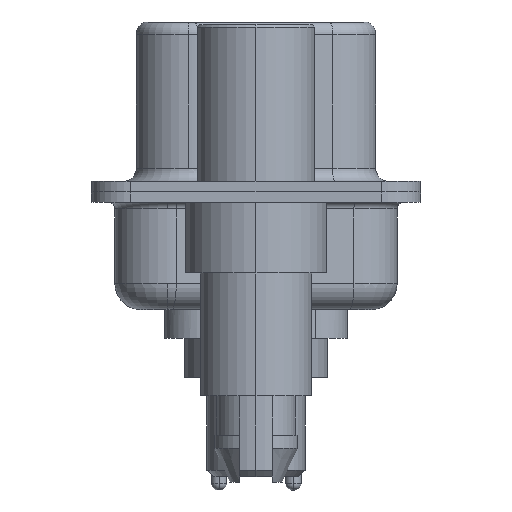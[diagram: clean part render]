
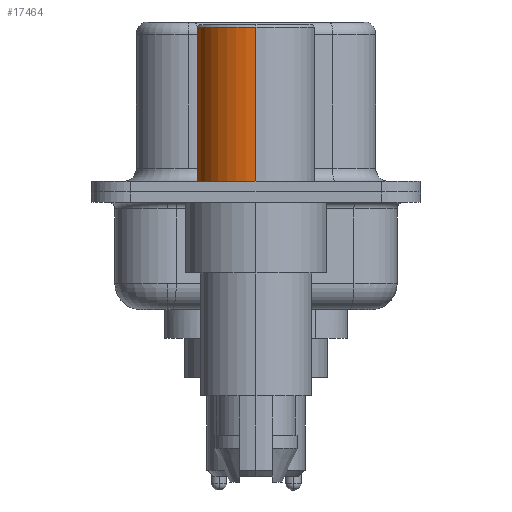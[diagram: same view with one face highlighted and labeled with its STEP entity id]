
A CAD part, left-side view. The second image highlights one B-rep face of the part: STEP entity #17464.
In plain terms, the highlighted cylindrical face has radius 2.25 mm (diameter 4.5 mm), a partial arc.
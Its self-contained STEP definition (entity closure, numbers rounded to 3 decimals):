
#1502 = EDGE_CURVE ( 'NONE', #6364, #8252, #3485, .T. ) ;
#1973 = CARTESIAN_POINT ( 'NONE',  ( 0., 0., 0.4 ) ) ;
#2702 = VECTOR ( 'NONE', #10057, 1000. ) ;
#3357 = CARTESIAN_POINT ( 'NONE',  ( -2.25, 0., 0.4 ) ) ;
#3378 = DIRECTION ( 'NONE',  ( 1., 0., 0. ) ) ;
#3485 = LINE ( 'NONE', #13438, #18408 ) ;
#3657 = CIRCLE ( 'NONE', #4676, 2.25 ) ;
#4417 = CARTESIAN_POINT ( 'NONE',  ( 0., 0., 6.3 ) ) ;
#4676 = AXIS2_PLACEMENT_3D ( 'NONE', #4417, #14560, #5862 ) ;
#4959 = EDGE_CURVE ( 'NONE', #15117, #11010, #6518, .T. ) ;
#5862 = DIRECTION ( 'NONE',  ( 1., 0., 0. ) ) ;
#6159 = CARTESIAN_POINT ( 'NONE',  ( 0., 0., 0.581 ) ) ;
#6364 = VERTEX_POINT ( 'NONE', #18380 ) ;
#6518 = LINE ( 'NONE', #13724, #2702 ) ;
#6620 = CARTESIAN_POINT ( 'NONE',  ( 2.25, 0., 6.3 ) ) ;
#7537 = CYLINDRICAL_SURFACE ( 'NONE', #13318, 2.25 ) ;
#7561 = AXIS2_PLACEMENT_3D ( 'NONE', #1973, #12103, #3378 ) ;
#8252 = VERTEX_POINT ( 'NONE', #6620 ) ;
#9093 = ORIENTED_EDGE ( 'NONE', *, *, #10716, .T. ) ;
#10057 = DIRECTION ( 'NONE',  ( 0., 0., 1. ) ) ;
#10716 = EDGE_CURVE ( 'NONE', #6364, #15117, #15681, .T. ) ;
#11003 = ORIENTED_EDGE ( 'NONE', *, *, #18572, .F. ) ;
#11010 = VERTEX_POINT ( 'NONE', #16993 ) ;
#12103 = DIRECTION ( 'NONE',  ( 0., 0., 1. ) ) ;
#12374 = ORIENTED_EDGE ( 'NONE', *, *, #1502, .F. ) ;
#13318 = AXIS2_PLACEMENT_3D ( 'NONE', #6159, #14662, #16290 ) ;
#13438 = CARTESIAN_POINT ( 'NONE',  ( 2.25, 0., 0.581 ) ) ;
#13724 = CARTESIAN_POINT ( 'NONE',  ( -2.25, 0., 0.581 ) ) ;
#14560 = DIRECTION ( 'NONE',  ( 0., 0., 1. ) ) ;
#14662 = DIRECTION ( 'NONE',  ( 0., 0., 1. ) ) ;
#15117 = VERTEX_POINT ( 'NONE', #3357 ) ;
#15240 = FACE_OUTER_BOUND ( 'NONE', #15654, .T. ) ;
#15654 = EDGE_LOOP ( 'NONE', ( #9093, #18207, #11003, #12374 ) ) ;
#15681 = CIRCLE ( 'NONE', #7561, 2.25 ) ;
#16290 = DIRECTION ( 'NONE',  ( 1., 0., 0. ) ) ;
#16492 = DIRECTION ( 'NONE',  ( 0., 0., 1. ) ) ;
#16993 = CARTESIAN_POINT ( 'NONE',  ( -2.25, 0., 6.3 ) ) ;
#17464 = ADVANCED_FACE ( 'NONE', ( #15240 ), #7537, .T. ) ;
#18207 = ORIENTED_EDGE ( 'NONE', *, *, #4959, .T. ) ;
#18380 = CARTESIAN_POINT ( 'NONE',  ( 2.25, 0., 0.4 ) ) ;
#18408 = VECTOR ( 'NONE', #16492, 1000. ) ;
#18572 = EDGE_CURVE ( 'NONE', #8252, #11010, #3657, .T. ) ;
